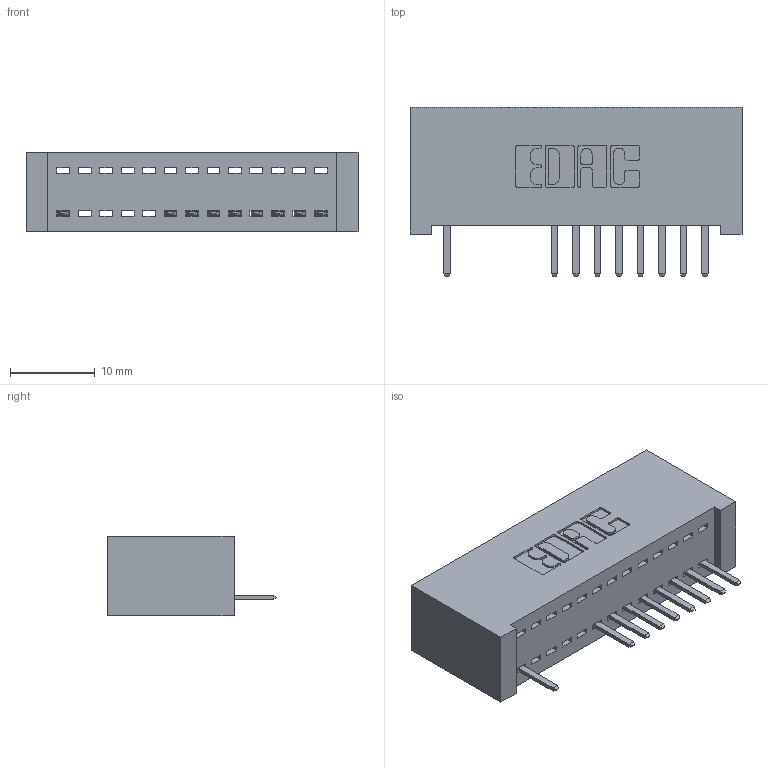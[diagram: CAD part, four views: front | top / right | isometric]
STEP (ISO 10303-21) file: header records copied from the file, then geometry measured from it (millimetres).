
FILE_DESCRIPTION (( 'STEP AP203' ), '1' );
FILE_NAME ('392-013-520-101.STEP', '2018-08-14T22:48:51', ( '' ), ( '' ), 'SwSTEP 2.0', 'SolidWorks 2016', '' );
FILE_SCHEMA (( 'CONFIG_CONTROL_DESIGN' ));
Length unit declared in the file: inch
Products named in the file (3): 345-292-001_345-293-120; 392-013-520-101; 342 Part_Lugless
Assembly tree (10 placements, depth 2):
  392-013-520-101
    342 Part_Lugless
    345-292-001_345-293-120  x9
Bounding box: 39.27 x 20.02 x 9.4 mm (x, y, z)
Volume: 3673.6 mm3; surface area: 4856.5 mm2
Topology: 10 solids, 10 shells, 708 faces, 2099 edges, 1374 vertices
Faces by surface type: plane 506, cylinder 202
Entity records: 11275 total; most frequent: CARTESIAN_POINT 1985, ORIENTED_EDGE 1926, DIRECTION 1709, EDGE_CURVE 963, VECTOR 839, LINE 839, VERTEX_POINT 638, AXIS2_PLACEMENT_3D 435
